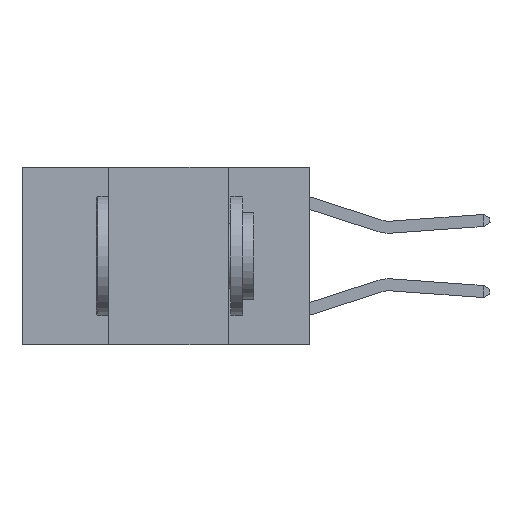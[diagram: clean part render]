
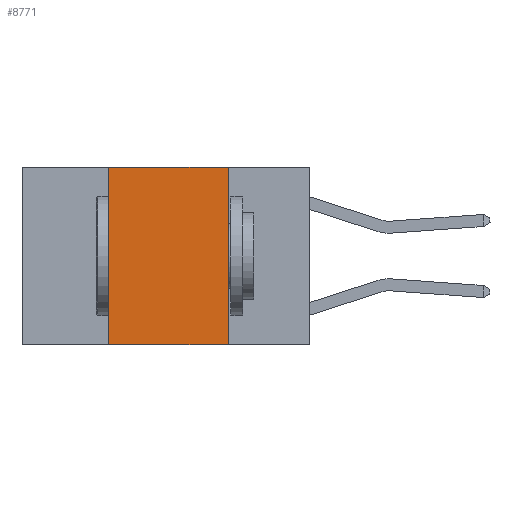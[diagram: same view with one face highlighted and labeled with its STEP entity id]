
A CAD part, left-side view. The second image highlights one B-rep face of the part: STEP entity #8771.
In plain terms, the highlighted planar face has unit normal (-1, 0, 0).
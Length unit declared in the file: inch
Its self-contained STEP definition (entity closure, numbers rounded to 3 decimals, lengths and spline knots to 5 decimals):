
#266 = LINE ( 'NONE', #5271, #2220 ) ;
#1327 = AXIS2_PLACEMENT_3D ( 'NONE', #12228, #7298, #3549 ) ;
#1498 = ORIENTED_EDGE ( 'NONE', *, *, #6320, .T. ) ;
#2220 = VECTOR ( 'NONE', #10326, 39.37008 ) ;
#2622 = CARTESIAN_POINT ( 'NONE',  ( 0., 0.6, 0. ) ) ;
#2787 = ORIENTED_EDGE ( 'NONE', *, *, #15132, .F. ) ;
#2835 = CARTESIAN_POINT ( 'NONE',  ( 0., 0.6, -0.37 ) ) ;
#3549 = DIRECTION ( 'NONE',  ( 0., 0., -1. ) ) ;
#3859 = VERTEX_POINT ( 'NONE', #13705 ) ;
#4077 = ORIENTED_EDGE ( 'NONE', *, *, #13652, .F. ) ;
#5269 = CARTESIAN_POINT ( 'NONE',  ( 0., 0.17, -0.37 ) ) ;
#5271 = CARTESIAN_POINT ( 'NONE',  ( 0., 0.42, 0. ) ) ;
#5373 = LINE ( 'NONE', #2835, #12365 ) ;
#5607 = VECTOR ( 'NONE', #14098, 39.37008 ) ;
#5646 = CARTESIAN_POINT ( 'NONE',  ( 0., 0.17, 0. ) ) ;
#5787 = EDGE_LOOP ( 'NONE', ( #5878, #4077, #2787, #1498 ) ) ;
#5878 = ORIENTED_EDGE ( 'NONE', *, *, #15933, .F. ) ;
#5916 = VERTEX_POINT ( 'NONE', #5269 ) ;
#5980 = LINE ( 'NONE', #5646, #12986 ) ;
#6320 = EDGE_CURVE ( 'NONE', #11640, #5916, #5373, .T. ) ;
#7298 = DIRECTION ( 'NONE',  ( 1., 0., 0. ) ) ;
#7865 = DIRECTION ( 'NONE',  ( 0., -1., 0. ) ) ;
#7887 = CARTESIAN_POINT ( 'NONE',  ( 0., 0.42, 0. ) ) ;
#8771 = ADVANCED_FACE ( 'NONE', ( #14711 ), #15028, .F. ) ;
#9781 = DIRECTION ( 'NONE',  ( 0., 0., -1. ) ) ;
#10326 = DIRECTION ( 'NONE',  ( 0., 0., 1. ) ) ;
#11640 = VERTEX_POINT ( 'NONE', #13455 ) ;
#12228 = CARTESIAN_POINT ( 'NONE',  ( 0., 0.6, 0. ) ) ;
#12365 = VECTOR ( 'NONE', #7865, 39.37008 ) ;
#12986 = VECTOR ( 'NONE', #9781, 39.37008 ) ;
#13008 = LINE ( 'NONE', #2622, #5607 ) ;
#13455 = CARTESIAN_POINT ( 'NONE',  ( 0., 0.42, -0.37 ) ) ;
#13652 = EDGE_CURVE ( 'NONE', #14682, #3859, #13008, .T. ) ;
#13705 = CARTESIAN_POINT ( 'NONE',  ( 0., 0.17, 0. ) ) ;
#14098 = DIRECTION ( 'NONE',  ( 0., -1., 0. ) ) ;
#14682 = VERTEX_POINT ( 'NONE', #7887 ) ;
#14711 = FACE_OUTER_BOUND ( 'NONE', #5787, .T. ) ;
#15028 = PLANE ( 'NONE',  #1327 ) ;
#15132 = EDGE_CURVE ( 'NONE', #11640, #14682, #266, .T. ) ;
#15933 = EDGE_CURVE ( 'NONE', #3859, #5916, #5980, .T. ) ;
